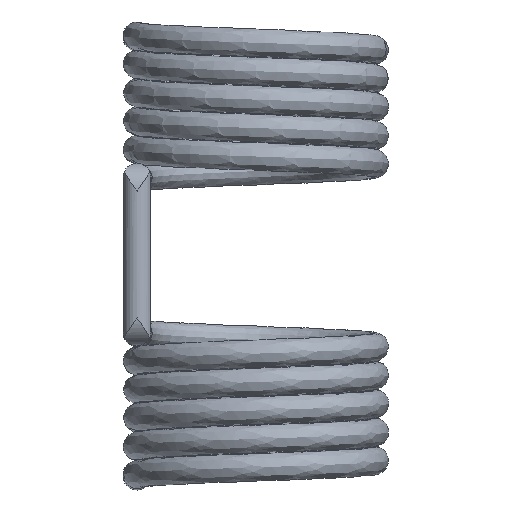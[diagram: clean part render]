
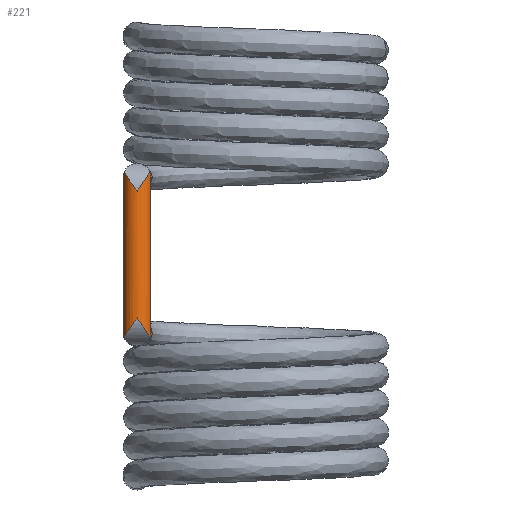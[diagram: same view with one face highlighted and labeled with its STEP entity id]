
A CAD part, top view. The second image highlights one B-rep face of the part: STEP entity #221.
In plain terms, the highlighted cylindrical face has radius 0.572 mm (diameter 1.143 mm), a full revolution.
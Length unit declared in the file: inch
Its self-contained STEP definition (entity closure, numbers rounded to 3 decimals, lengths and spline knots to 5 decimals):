
#29=FACE_BOUND('',#61,.T.);
#42=ELLIPSE('',#253,0.03182,0.0225);
#43=ELLIPSE('',#254,0.03182,0.0225);
#44=ELLIPSE('',#255,0.03182,0.0225);
#45=ELLIPSE('',#256,0.03182,0.0225);
#46=ELLIPSE('',#257,0.03182,0.0225);
#47=ELLIPSE('',#258,0.03182,0.0225);
#49=FACE_OUTER_BOUND('',#60,.T.);
#60=EDGE_LOOP('',(#157,#158,#159,#160,#161));
#61=EDGE_LOOP('',(#162,#163,#164,#165,#166));
#83=B_SPLINE_CURVE_WITH_KNOTS('',3,(#332,#333,#334,#335,#336,#337,#338,
#339),.UNSPECIFIED.,.F.,.F.,(4,2,2,4),(0.33449,0.35726,
0.39528,0.4333),.UNSPECIFIED.);
#84=B_SPLINE_CURVE_WITH_KNOTS('',3,(#341,#342,#343,#344,#345,#346,#347,
#348),.UNSPECIFIED.,.F.,.F.,(4,2,2,4),(0.,0.03802,0.07604,
0.09881),.UNSPECIFIED.);
#87=B_SPLINE_CURVE_WITH_KNOTS('',3,(#373,#374,#375,#376,#377,#378,#379,
#380),.UNSPECIFIED.,.F.,.F.,(4,2,2,4),(0.,0.03802,0.07604,
0.09881),.UNSPECIFIED.);
#88=B_SPLINE_CURVE_WITH_KNOTS('',3,(#382,#383,#384,#385,#386,#387,#388,
#389),.UNSPECIFIED.,.F.,.F.,(4,2,2,4),(0.33449,0.35726,
0.39528,0.4333),.UNSPECIFIED.);
#97=VERTEX_POINT('',#330);
#98=VERTEX_POINT('',#331);
#99=VERTEX_POINT('',#340);
#101=VERTEX_POINT('',#367);
#102=VERTEX_POINT('',#368);
#103=VERTEX_POINT('',#370);
#104=VERTEX_POINT('',#372);
#105=VERTEX_POINT('',#381);
#106=VERTEX_POINT('',#391);
#107=VERTEX_POINT('',#392);
#123=EDGE_CURVE('',#97,#98,#83,.T.);
#124=EDGE_CURVE('',#98,#99,#84,.T.);
#127=EDGE_CURVE('',#101,#102,#42,.T.);
#128=EDGE_CURVE('',#103,#101,#43,.T.);
#129=EDGE_CURVE('',#104,#103,#87,.T.);
#130=EDGE_CURVE('',#105,#104,#88,.T.);
#131=EDGE_CURVE('',#102,#105,#44,.T.);
#132=EDGE_CURVE('',#106,#107,#45,.T.);
#133=EDGE_CURVE('',#99,#107,#46,.T.);
#134=EDGE_CURVE('',#106,#97,#47,.T.);
#157=ORIENTED_EDGE('',*,*,#127,.F.);
#158=ORIENTED_EDGE('',*,*,#128,.F.);
#159=ORIENTED_EDGE('',*,*,#129,.F.);
#160=ORIENTED_EDGE('',*,*,#130,.F.);
#161=ORIENTED_EDGE('',*,*,#131,.F.);
#162=ORIENTED_EDGE('',*,*,#132,.T.);
#163=ORIENTED_EDGE('',*,*,#133,.F.);
#164=ORIENTED_EDGE('',*,*,#124,.F.);
#165=ORIENTED_EDGE('',*,*,#123,.F.);
#166=ORIENTED_EDGE('',*,*,#134,.F.);
#214=CYLINDRICAL_SURFACE('',#252,0.0225);
#221=ADVANCED_FACE('',(#49,#29),#214,.T.);
#252=AXIS2_PLACEMENT_3D('',#366,#280,#281);
#253=AXIS2_PLACEMENT_3D('',#369,#282,#283);
#254=AXIS2_PLACEMENT_3D('',#371,#284,#285);
#255=AXIS2_PLACEMENT_3D('',#390,#286,#287);
#256=AXIS2_PLACEMENT_3D('',#393,#288,#289);
#257=AXIS2_PLACEMENT_3D('',#394,#290,#291);
#258=AXIS2_PLACEMENT_3D('',#395,#292,#293);
#280=DIRECTION('center_axis',(0.,1.,0.));
#281=DIRECTION('ref_axis',(1.,0.,0.));
#282=DIRECTION('center_axis',(0.,-0.707,-0.707));
#283=DIRECTION('ref_axis',(0.,0.707,-0.707));
#284=DIRECTION('center_axis',(0.,-0.707,-0.707));
#285=DIRECTION('ref_axis',(0.,0.707,-0.707));
#286=DIRECTION('center_axis',(0.,-0.707,-0.707));
#287=DIRECTION('ref_axis',(0.,0.707,-0.707));
#288=DIRECTION('center_axis',(0.,-0.707,0.707));
#289=DIRECTION('ref_axis',(0.,-0.707,-0.707));
#290=DIRECTION('center_axis',(0.,0.707,-0.707));
#291=DIRECTION('ref_axis',(0.,-0.707,-0.707));
#292=DIRECTION('center_axis',(0.,0.707,-0.707));
#293=DIRECTION('ref_axis',(0.,-0.707,-0.707));
#330=CARTESIAN_POINT('',(-0.02048,0.48932,0.68682));
#331=CARTESIAN_POINT('',(0.,0.4575,0.7));
#332=CARTESIAN_POINT('Ctrl Pts',(-0.02048,0.48932,
0.68682));
#333=CARTESIAN_POINT('Ctrl Pts',(-0.0195,0.48716,0.68898));
#334=CARTESIAN_POINT('Ctrl Pts',(-0.01822,0.48484,
0.69085));
#335=CARTESIAN_POINT('Ctrl Pts',(-0.01471,0.47889,
0.69484));
#336=CARTESIAN_POINT('Ctrl Pts',(-0.01194,0.47467,0.69684));
#337=CARTESIAN_POINT('Ctrl Pts',(-0.00602,0.46601,
0.69942));
#338=CARTESIAN_POINT('Ctrl Pts',(-0.00288,0.46157,
0.7));
#339=CARTESIAN_POINT('Ctrl Pts',(0.,0.4575,0.7));
#340=CARTESIAN_POINT('',(0.02048,0.48932,0.68682));
#341=CARTESIAN_POINT('Ctrl Pts',(0.,0.4575,0.7));
#342=CARTESIAN_POINT('Ctrl Pts',(0.00288,0.46157,
0.7));
#343=CARTESIAN_POINT('Ctrl Pts',(0.00602,0.46601,0.69942));
#344=CARTESIAN_POINT('Ctrl Pts',(0.01194,0.47467,0.69684));
#345=CARTESIAN_POINT('Ctrl Pts',(0.01471,0.47889,0.69484));
#346=CARTESIAN_POINT('Ctrl Pts',(0.01822,0.48484,0.69085));
#347=CARTESIAN_POINT('Ctrl Pts',(0.0195,0.48716,0.68898));
#348=CARTESIAN_POINT('Ctrl Pts',(0.02048,0.48932,0.68682));
#366=CARTESIAN_POINT('Origin',(0.,0.,0.6775));
#367=CARTESIAN_POINT('',(-0.0225,0.23,0.6775));
#368=CARTESIAN_POINT('',(0.0225,0.23,0.6775));
#369=CARTESIAN_POINT('Origin',(0.,0.23,0.6775));
#370=CARTESIAN_POINT('',(-0.02048,0.22068,0.68682));
#371=CARTESIAN_POINT('Origin',(0.,0.23,0.6775));
#372=CARTESIAN_POINT('',(0.,0.2525,0.7));
#373=CARTESIAN_POINT('Ctrl Pts',(0.,0.2525,0.7));
#374=CARTESIAN_POINT('Ctrl Pts',(-0.00288,0.24843,
0.7));
#375=CARTESIAN_POINT('Ctrl Pts',(-0.00602,0.24399,
0.69942));
#376=CARTESIAN_POINT('Ctrl Pts',(-0.01194,0.23533,0.69684));
#377=CARTESIAN_POINT('Ctrl Pts',(-0.01471,0.23111,
0.69484));
#378=CARTESIAN_POINT('Ctrl Pts',(-0.01822,0.22516,
0.69085));
#379=CARTESIAN_POINT('Ctrl Pts',(-0.0195,0.22284,0.68898));
#380=CARTESIAN_POINT('Ctrl Pts',(-0.02048,0.22068,
0.68682));
#381=CARTESIAN_POINT('',(0.02048,0.22068,0.68682));
#382=CARTESIAN_POINT('Ctrl Pts',(0.02048,0.22068,0.68682));
#383=CARTESIAN_POINT('Ctrl Pts',(0.0195,0.22284,0.68898));
#384=CARTESIAN_POINT('Ctrl Pts',(0.01822,0.22516,0.69085));
#385=CARTESIAN_POINT('Ctrl Pts',(0.01471,0.23111,0.69484));
#386=CARTESIAN_POINT('Ctrl Pts',(0.01194,0.23533,0.69684));
#387=CARTESIAN_POINT('Ctrl Pts',(0.00602,0.24399,0.69942));
#388=CARTESIAN_POINT('Ctrl Pts',(0.00288,0.24843,
0.7));
#389=CARTESIAN_POINT('Ctrl Pts',(0.,0.2525,0.7));
#390=CARTESIAN_POINT('Origin',(0.,0.23,0.6775));
#391=CARTESIAN_POINT('',(-0.0225,0.48,0.6775));
#392=CARTESIAN_POINT('',(0.0225,0.48,0.6775));
#393=CARTESIAN_POINT('Origin',(0.,0.48,0.6775));
#394=CARTESIAN_POINT('Origin',(0.,0.48,0.6775));
#395=CARTESIAN_POINT('Origin',(0.,0.48,0.6775));
